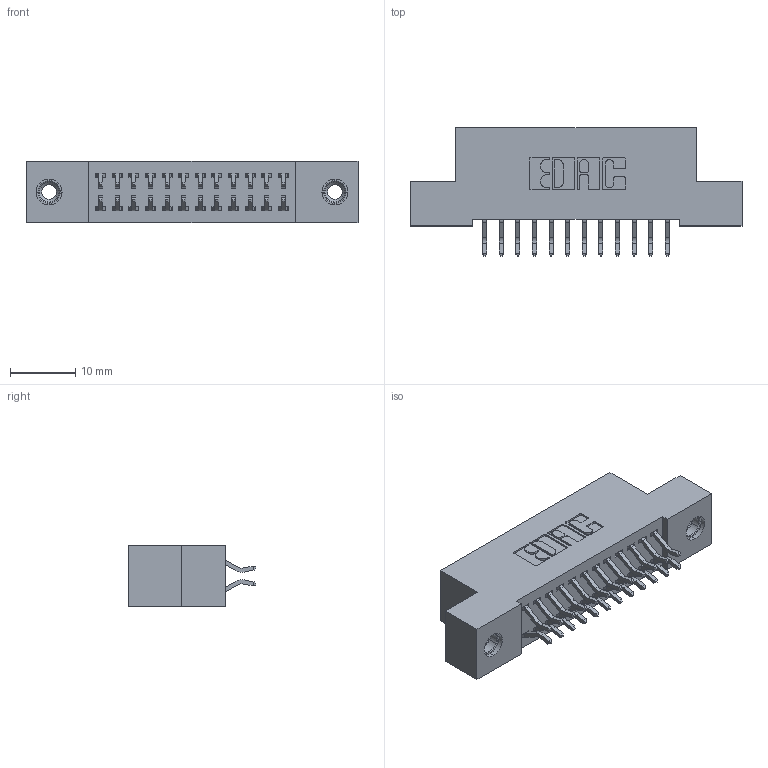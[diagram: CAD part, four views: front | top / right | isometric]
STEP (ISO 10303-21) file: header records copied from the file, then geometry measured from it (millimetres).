
FILE_DESCRIPTION (( 'STEP AP203' ), '1' );
FILE_NAME ('342-024-556-208.STEP', '2018-08-11T02:53:12', ( '' ), ( '' ), 'SwSTEP 2.0', 'SolidWorks 2016', '' );
FILE_SCHEMA (( 'CONFIG_CONTROL_DESIGN' ));
Length unit declared in the file: inch
Products named in the file (4): 345-292-001_556 Tail; 345-250-001_345-250-003-102; 342-024-556-208; 342 Part_TI
Assembly tree (27 placements, depth 2):
  342-024-556-208
    342 Part_TI
    345-292-001_556 Tail  x24
    345-250-001_345-250-003-102  x2
Bounding box: 50.8 x 19.58 x 9.4 mm (x, y, z)
Volume: 4416.1 mm3; surface area: 6436.1 mm2
Topology: 27 solids, 27 shells, 1562 faces, 4587 edges, 3018 vertices
Faces by surface type: plane 1058, cylinder 488, cone 12, torus 4
Entity records: 12874 total; most frequent: CARTESIAN_POINT 2165, ORIENTED_EDGE 2082, DIRECTION 1923, EDGE_CURVE 1041, VECTOR 885, LINE 885, VERTEX_POINT 688, AXIS2_PLACEMENT_3D 519
